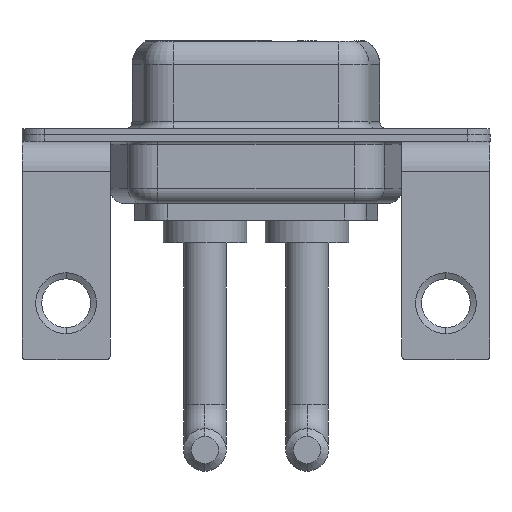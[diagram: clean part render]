
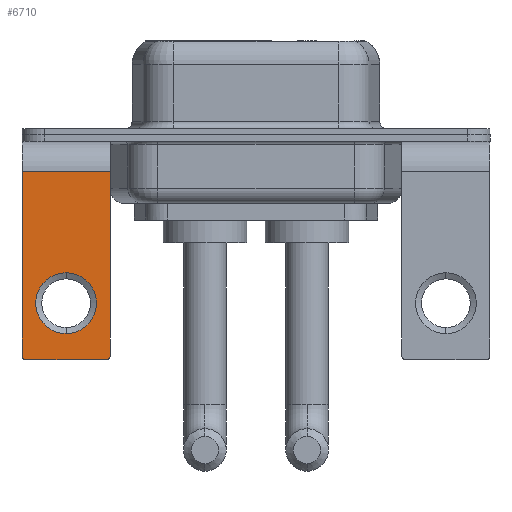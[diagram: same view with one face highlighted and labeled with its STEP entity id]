
A CAD part, front view. The second image highlights one B-rep face of the part: STEP entity #6710.
In plain terms, the highlighted planar face has unit normal (0, -1, 0).
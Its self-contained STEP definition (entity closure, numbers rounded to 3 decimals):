
#107 = DIRECTION ( 'NONE',  ( 0., 1., 0. ) ) ;
#344 = EDGE_CURVE ( 'NONE', #4253, #6823, #9200, .T. ) ;
#363 = VERTEX_POINT ( 'NONE', #9135 ) ;
#584 = VECTOR ( 'NONE', #11437, 1000. ) ;
#641 = AXIS2_PLACEMENT_3D ( 'NONE', #1891, #107, #1761 ) ;
#1147 = DIRECTION ( 'NONE',  ( 0., 1., 0. ) ) ;
#1450 = DIRECTION ( 'NONE',  ( 0., -1., 0. ) ) ;
#1761 = DIRECTION ( 'NONE',  ( 0., 0., 1. ) ) ;
#1891 = CARTESIAN_POINT ( 'NONE',  ( 2.9, -6.25, -2.4 ) ) ;
#2097 = CARTESIAN_POINT ( 'NONE',  ( 0., -6.25, -11.07 ) ) ;
#2177 = AXIS2_PLACEMENT_3D ( 'NONE', #13003, #1147, #2437 ) ;
#2186 = DIRECTION ( 'NONE',  ( 0., 0., 1. ) ) ;
#2217 = EDGE_LOOP ( 'NONE', ( #7678, #2430, #3204, #8392, #13543, #2684 ) ) ;
#2219 = EDGE_LOOP ( 'NONE', ( #7306, #6912 ) ) ;
#2239 = FACE_OUTER_BOUND ( 'NONE', #2217, .T. ) ;
#2402 = AXIS2_PLACEMENT_3D ( 'NONE', #10274, #1450, #2588 ) ;
#2426 = EDGE_CURVE ( 'NONE', #13400, #13376, #13126, .T. ) ;
#2430 = ORIENTED_EDGE ( 'NONE', *, *, #11336, .T. ) ;
#2437 = DIRECTION ( 'NONE',  ( 0., 0., 1. ) ) ;
#2524 = CARTESIAN_POINT ( 'NONE',  ( 0., -6.25, -13.07 ) ) ;
#2588 = DIRECTION ( 'NONE',  ( 0., 0., 1. ) ) ;
#2684 = ORIENTED_EDGE ( 'NONE', *, *, #9914, .T. ) ;
#3074 = CIRCLE ( 'NONE', #2402, 0.25 ) ;
#3204 = ORIENTED_EDGE ( 'NONE', *, *, #344, .F. ) ;
#4253 = VERTEX_POINT ( 'NONE', #7300 ) ;
#4716 = LINE ( 'NONE', #7911, #8448 ) ;
#5120 = CIRCLE ( 'NONE', #6941, 0.25 ) ;
#5796 = DIRECTION ( 'NONE',  ( -1., 0., 0. ) ) ;
#5873 = CARTESIAN_POINT ( 'NONE',  ( -2.65, -6.25, -14.8 ) ) ;
#6156 = VERTEX_POINT ( 'NONE', #13884 ) ;
#6184 = FACE_BOUND ( 'NONE', #2219, .T. ) ;
#6298 = LINE ( 'NONE', #9559, #8990 ) ;
#6591 = PLANE ( 'NONE',  #641 ) ;
#6710 = ADVANCED_FACE ( 'NONE', ( #6184, #2239 ), #6591, .F. ) ;
#6823 = VERTEX_POINT ( 'NONE', #5873 ) ;
#6912 = ORIENTED_EDGE ( 'NONE', *, *, #11300, .T. ) ;
#6941 = AXIS2_PLACEMENT_3D ( 'NONE', #13947, #11953, #2186 ) ;
#6952 = AXIS2_PLACEMENT_3D ( 'NONE', #2097, #9638, #8726 ) ;
#7061 = CARTESIAN_POINT ( 'NONE',  ( -2.9, -6.25, -14.55 ) ) ;
#7174 = CIRCLE ( 'NONE', #6952, 2. ) ;
#7300 = CARTESIAN_POINT ( 'NONE',  ( 2.65, -6.25, -14.8 ) ) ;
#7306 = ORIENTED_EDGE ( 'NONE', *, *, #2426, .T. ) ;
#7678 = ORIENTED_EDGE ( 'NONE', *, *, #13593, .T. ) ;
#7843 = VECTOR ( 'NONE', #10264, 1000. ) ;
#7911 = CARTESIAN_POINT ( 'NONE',  ( 2.9, -6.25, -2.4 ) ) ;
#7994 = CARTESIAN_POINT ( 'NONE',  ( -2.9, -6.25, -2.4 ) ) ;
#8392 = ORIENTED_EDGE ( 'NONE', *, *, #12855, .T. ) ;
#8448 = VECTOR ( 'NONE', #5796, 1000. ) ;
#8726 = DIRECTION ( 'NONE',  ( 0., 0., 1. ) ) ;
#8764 = VERTEX_POINT ( 'NONE', #10534 ) ;
#8990 = VECTOR ( 'NONE', #10490, 1000. ) ;
#9074 = LINE ( 'NONE', #7994, #584 ) ;
#9135 = CARTESIAN_POINT ( 'NONE',  ( 2.9, -6.25, -2.4 ) ) ;
#9200 = LINE ( 'NONE', #10410, #7843 ) ;
#9559 = CARTESIAN_POINT ( 'NONE',  ( 2.9, -6.25, -2.4 ) ) ;
#9638 = DIRECTION ( 'NONE',  ( 0., 1., 0. ) ) ;
#9914 = EDGE_CURVE ( 'NONE', #363, #8764, #4716, .T. ) ;
#10086 = VERTEX_POINT ( 'NONE', #7061 ) ;
#10264 = DIRECTION ( 'NONE',  ( -1., 0., 0. ) ) ;
#10274 = CARTESIAN_POINT ( 'NONE',  ( -2.65, -6.25, -14.55 ) ) ;
#10410 = CARTESIAN_POINT ( 'NONE',  ( 2.9, -6.25, -14.8 ) ) ;
#10490 = DIRECTION ( 'NONE',  ( 0., 0., -1. ) ) ;
#10534 = CARTESIAN_POINT ( 'NONE',  ( -2.9, -6.25, -2.4 ) ) ;
#11300 = EDGE_CURVE ( 'NONE', #13376, #13400, #7174, .T. ) ;
#11336 = EDGE_CURVE ( 'NONE', #10086, #6823, #3074, .T. ) ;
#11437 = DIRECTION ( 'NONE',  ( 0., 0., -1. ) ) ;
#11475 = EDGE_CURVE ( 'NONE', #363, #6156, #6298, .T. ) ;
#11953 = DIRECTION ( 'NONE',  ( 0., -1., 0. ) ) ;
#12855 = EDGE_CURVE ( 'NONE', #4253, #6156, #5120, .T. ) ;
#13003 = CARTESIAN_POINT ( 'NONE',  ( 0., -6.25, -11.07 ) ) ;
#13126 = CIRCLE ( 'NONE', #2177, 2. ) ;
#13236 = CARTESIAN_POINT ( 'NONE',  ( 0., -6.25, -9.07 ) ) ;
#13376 = VERTEX_POINT ( 'NONE', #13236 ) ;
#13400 = VERTEX_POINT ( 'NONE', #2524 ) ;
#13543 = ORIENTED_EDGE ( 'NONE', *, *, #11475, .F. ) ;
#13593 = EDGE_CURVE ( 'NONE', #8764, #10086, #9074, .T. ) ;
#13884 = CARTESIAN_POINT ( 'NONE',  ( 2.9, -6.25, -14.55 ) ) ;
#13947 = CARTESIAN_POINT ( 'NONE',  ( 2.65, -6.25, -14.55 ) ) ;
